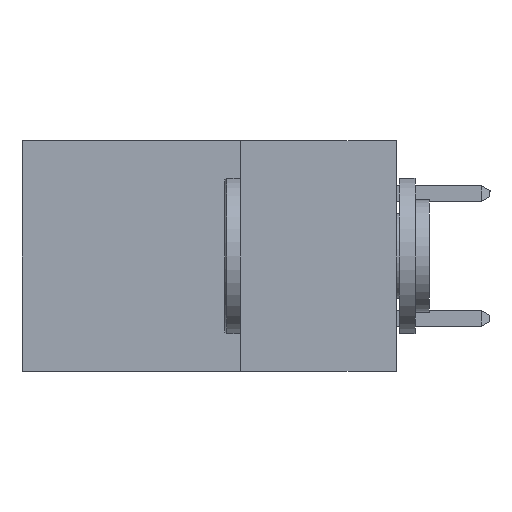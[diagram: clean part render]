
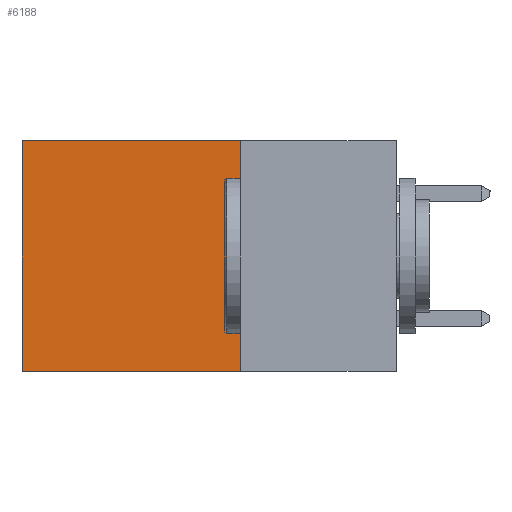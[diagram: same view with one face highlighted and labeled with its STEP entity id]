
A CAD part, left-side view. The second image highlights one B-rep face of the part: STEP entity #6188.
In plain terms, the highlighted planar face has unit normal (-1, 0, 0).
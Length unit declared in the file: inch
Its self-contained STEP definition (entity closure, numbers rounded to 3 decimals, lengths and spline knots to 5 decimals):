
#178 = LINE ( 'NONE', #15524, #1152 ) ;
#1152 = VECTOR ( 'NONE', #7265, 39.37008 ) ;
#1290 = LINE ( 'NONE', #4120, #13335 ) ;
#2067 = PLANE ( 'NONE',  #11919 ) ;
#2239 = LINE ( 'NONE', #7786, #12217 ) ;
#2601 = DIRECTION ( 'NONE',  ( 0., 1., 0. ) ) ;
#2702 = VECTOR ( 'NONE', #6535, 39.37008 ) ;
#3317 = VERTEX_POINT ( 'NONE', #3899 ) ;
#3649 = EDGE_LOOP ( 'NONE', ( #16225, #14197, #14452, #5486 ) ) ;
#3899 = CARTESIAN_POINT ( 'NONE',  ( 0.2615, 0.25, 0. ) ) ;
#4120 = CARTESIAN_POINT ( 'NONE',  ( 0.2615, 0.25, -0.37 ) ) ;
#4296 = EDGE_CURVE ( 'NONE', #3317, #14401, #1290, .T. ) ;
#4799 = CARTESIAN_POINT ( 'NONE',  ( 0.2615, 0.25, -0.37 ) ) ;
#4850 = EDGE_CURVE ( 'NONE', #17257, #8944, #178, .T. ) ;
#5486 = ORIENTED_EDGE ( 'NONE', *, *, #6310, .T. ) ;
#6188 = ADVANCED_FACE ( 'NONE', ( #6343 ), #2067, .F. ) ;
#6310 = EDGE_CURVE ( 'NONE', #3317, #17257, #2239, .T. ) ;
#6343 = FACE_OUTER_BOUND ( 'NONE', #3649, .T. ) ;
#6535 = DIRECTION ( 'NONE',  ( 0., 1., 0. ) ) ;
#7265 = DIRECTION ( 'NONE',  ( 0., 0., -1. ) ) ;
#7786 = CARTESIAN_POINT ( 'NONE',  ( 0.2615, 0.25, 0. ) ) ;
#8790 = DIRECTION ( 'NONE',  ( 1., 0., 0. ) ) ;
#8944 = VERTEX_POINT ( 'NONE', #16263 ) ;
#11260 = CARTESIAN_POINT ( 'NONE',  ( 0.2615, 0.6, 0. ) ) ;
#11390 = EDGE_CURVE ( 'NONE', #14401, #8944, #11982, .T. ) ;
#11919 = AXIS2_PLACEMENT_3D ( 'NONE', #17430, #8790, #15791 ) ;
#11982 = LINE ( 'NONE', #16157, #2702 ) ;
#12217 = VECTOR ( 'NONE', #2601, 39.37008 ) ;
#13335 = VECTOR ( 'NONE', #15006, 39.37008 ) ;
#14197 = ORIENTED_EDGE ( 'NONE', *, *, #11390, .F. ) ;
#14401 = VERTEX_POINT ( 'NONE', #4799 ) ;
#14452 = ORIENTED_EDGE ( 'NONE', *, *, #4296, .F. ) ;
#15006 = DIRECTION ( 'NONE',  ( 0., 0., -1. ) ) ;
#15524 = CARTESIAN_POINT ( 'NONE',  ( 0.2615, 0.6, -0.37 ) ) ;
#15791 = DIRECTION ( 'NONE',  ( 0., 0., -1. ) ) ;
#16157 = CARTESIAN_POINT ( 'NONE',  ( 0.2615, 0.25, -0.37 ) ) ;
#16225 = ORIENTED_EDGE ( 'NONE', *, *, #4850, .T. ) ;
#16263 = CARTESIAN_POINT ( 'NONE',  ( 0.2615, 0.6, -0.37 ) ) ;
#17257 = VERTEX_POINT ( 'NONE', #11260 ) ;
#17430 = CARTESIAN_POINT ( 'NONE',  ( 0.2615, 0.25, -0.37 ) ) ;
